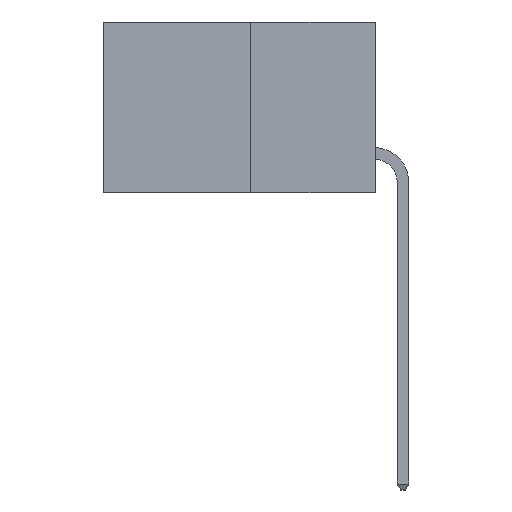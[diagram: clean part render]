
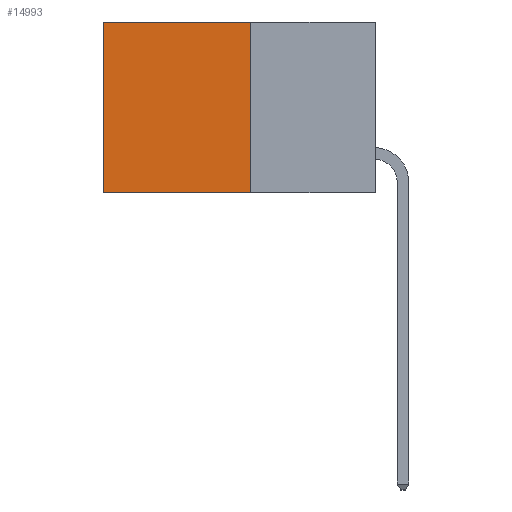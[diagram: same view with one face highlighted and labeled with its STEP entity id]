
A CAD part, left-side view. The second image highlights one B-rep face of the part: STEP entity #14993.
In plain terms, the highlighted planar face has unit normal (-1, 0, 0).
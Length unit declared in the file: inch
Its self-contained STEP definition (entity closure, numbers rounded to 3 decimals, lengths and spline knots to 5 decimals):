
#556 = CARTESIAN_POINT ( 'NONE',  ( 0.277, 0.27, -0.37 ) ) ;
#1833 = CARTESIAN_POINT ( 'NONE',  ( 0.277, 0.59, -0.37 ) ) ;
#2673 = ORIENTED_EDGE ( 'NONE', *, *, #3096, .T. ) ;
#2861 = VERTEX_POINT ( 'NONE', #1833 ) ;
#3096 = EDGE_CURVE ( 'NONE', #13774, #2861, #18274, .T. ) ;
#3913 = LINE ( 'NONE', #4609, #26834 ) ;
#4268 = EDGE_CURVE ( 'NONE', #9763, #13774, #3913, .T. ) ;
#4609 = CARTESIAN_POINT ( 'NONE',  ( 0.277, 0.27, 0. ) ) ;
#5051 = EDGE_CURVE ( 'NONE', #27230, #2861, #18197, .T. ) ;
#7617 = VECTOR ( 'NONE', #25258, 39.37008 ) ;
#9394 = DIRECTION ( 'NONE',  ( 0., 1., 0. ) ) ;
#9507 = FACE_OUTER_BOUND ( 'NONE', #21247, .T. ) ;
#9692 = CARTESIAN_POINT ( 'NONE',  ( 0.277, 0.27, -0.37 ) ) ;
#9763 = VERTEX_POINT ( 'NONE', #25546 ) ;
#10875 = ORIENTED_EDGE ( 'NONE', *, *, #4268, .T. ) ;
#11288 = DIRECTION ( 'NONE',  ( 0., 1., 0. ) ) ;
#12247 = VECTOR ( 'NONE', #9394, 39.37008 ) ;
#12840 = LINE ( 'NONE', #9692, #7617 ) ;
#13774 = VERTEX_POINT ( 'NONE', #22124 ) ;
#14774 = PLANE ( 'NONE',  #25635 ) ;
#14872 = DIRECTION ( 'NONE',  ( 0., 0., -1. ) ) ;
#14993 = ADVANCED_FACE ( 'NONE', ( #9507 ), #14774, .F. ) ;
#17163 = ORIENTED_EDGE ( 'NONE', *, *, #17399, .F. ) ;
#17399 = EDGE_CURVE ( 'NONE', #9763, #27230, #12840, .T. ) ;
#17572 = VECTOR ( 'NONE', #18187, 39.37008 ) ;
#18187 = DIRECTION ( 'NONE',  ( 0., 0., -1. ) ) ;
#18197 = LINE ( 'NONE', #24866, #12247 ) ;
#18274 = LINE ( 'NONE', #26965, #17572 ) ;
#21247 = EDGE_LOOP ( 'NONE', ( #2673, #24618, #17163, #10875 ) ) ;
#21569 = CARTESIAN_POINT ( 'NONE',  ( 0.277, 0.27, -0.37 ) ) ;
#22124 = CARTESIAN_POINT ( 'NONE',  ( 0.277, 0.59, 0. ) ) ;
#24618 = ORIENTED_EDGE ( 'NONE', *, *, #5051, .F. ) ;
#24866 = CARTESIAN_POINT ( 'NONE',  ( 0.277, 0.27, -0.37 ) ) ;
#25258 = DIRECTION ( 'NONE',  ( 0., 0., -1. ) ) ;
#25546 = CARTESIAN_POINT ( 'NONE',  ( 0.277, 0.27, 0. ) ) ;
#25635 = AXIS2_PLACEMENT_3D ( 'NONE', #21569, #28152, #14872 ) ;
#26834 = VECTOR ( 'NONE', #11288, 39.37008 ) ;
#26965 = CARTESIAN_POINT ( 'NONE',  ( 0.277, 0.59, -0.37 ) ) ;
#27230 = VERTEX_POINT ( 'NONE', #556 ) ;
#28152 = DIRECTION ( 'NONE',  ( 1., 0., 0. ) ) ;
